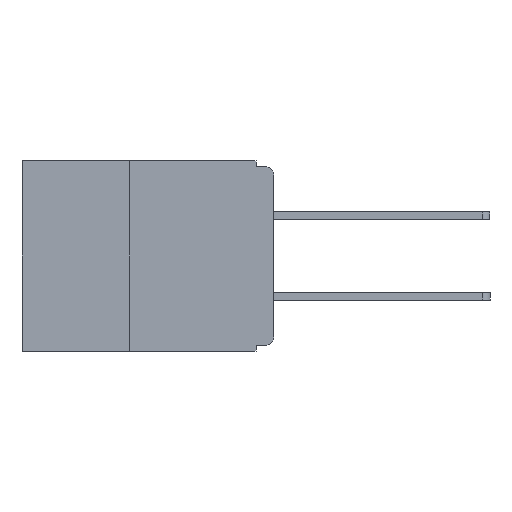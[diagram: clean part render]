
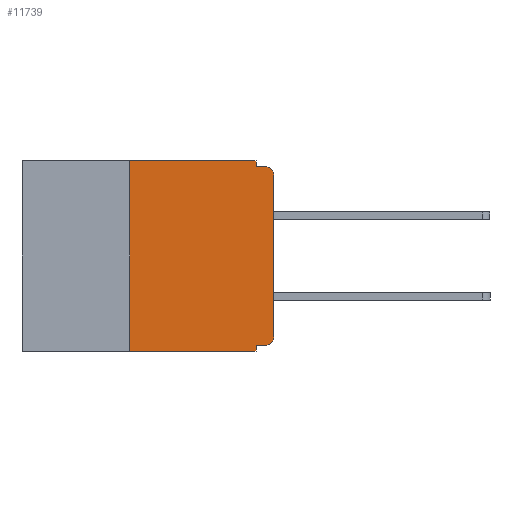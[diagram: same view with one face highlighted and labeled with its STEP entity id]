
A CAD part, left-side view. The second image highlights one B-rep face of the part: STEP entity #11739.
In plain terms, the highlighted planar face has unit normal (-1, 0, 0).
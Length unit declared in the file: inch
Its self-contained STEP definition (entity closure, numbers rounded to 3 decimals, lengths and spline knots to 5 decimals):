
#386 = CARTESIAN_POINT ( 'NONE',  ( 0., 0., -0.305 ) ) ;
#990 = VERTEX_POINT ( 'NONE', #12404 ) ;
#1145 = VERTEX_POINT ( 'NONE', #3089 ) ;
#1475 = LINE ( 'NONE', #6721, #4894 ) ;
#1728 = ORIENTED_EDGE ( 'NONE', *, *, #4678, .T. ) ;
#1759 = EDGE_CURVE ( 'NONE', #8024, #1145, #12991, .T. ) ;
#1938 = EDGE_CURVE ( 'NONE', #990, #3292, #2088, .T. ) ;
#2088 = LINE ( 'NONE', #8318, #7469 ) ;
#2094 = ORIENTED_EDGE ( 'NONE', *, *, #13673, .T. ) ;
#2218 = LINE ( 'NONE', #14178, #7942 ) ;
#2432 = ORIENTED_EDGE ( 'NONE', *, *, #4056, .F. ) ;
#2573 = CARTESIAN_POINT ( 'NONE',  ( 0., 0.437, 0. ) ) ;
#2944 = DIRECTION ( 'NONE',  ( -1., 0., 0. ) ) ;
#2991 = ORIENTED_EDGE ( 'NONE', *, *, #1938, .F. ) ;
#3089 = CARTESIAN_POINT ( 'NONE',  ( 0., 0.031, -0.33 ) ) ;
#3232 = CARTESIAN_POINT ( 'NONE',  ( 0., 0.015, -0.305 ) ) ;
#3292 = VERTEX_POINT ( 'NONE', #6554 ) ;
#3412 = ORIENTED_EDGE ( 'NONE', *, *, #3512, .F. ) ;
#3512 = EDGE_CURVE ( 'NONE', #6207, #990, #2218, .T. ) ;
#3688 = EDGE_CURVE ( 'NONE', #4758, #1145, #11585, .T. ) ;
#3736 = DIRECTION ( 'NONE',  ( 0., 0., -1. ) ) ;
#3903 = VECTOR ( 'NONE', #8673, 39.37008 ) ;
#4056 = EDGE_CURVE ( 'NONE', #3292, #9083, #5090, .T. ) ;
#4080 = AXIS2_PLACEMENT_3D ( 'NONE', #9697, #2944, #10752 ) ;
#4146 = ORIENTED_EDGE ( 'NONE', *, *, #6434, .F. ) ;
#4300 = AXIS2_PLACEMENT_3D ( 'NONE', #3232, #11186, #4588 ) ;
#4315 = CARTESIAN_POINT ( 'NONE',  ( 0., 0.437, -0.33 ) ) ;
#4477 = ORIENTED_EDGE ( 'NONE', *, *, #1759, .T. ) ;
#4588 = DIRECTION ( 'NONE',  ( 0., 0., -1. ) ) ;
#4678 = EDGE_CURVE ( 'NONE', #6570, #8162, #1475, .T. ) ;
#4758 = VERTEX_POINT ( 'NONE', #6008 ) ;
#4894 = VECTOR ( 'NONE', #6567, 39.37008 ) ;
#5090 = LINE ( 'NONE', #11175, #10291 ) ;
#5576 = ORIENTED_EDGE ( 'NONE', *, *, #3688, .F. ) ;
#5739 = ORIENTED_EDGE ( 'NONE', *, *, #8268, .F. ) ;
#5898 = CARTESIAN_POINT ( 'NONE',  ( 0., 0., -0.32 ) ) ;
#6008 = CARTESIAN_POINT ( 'NONE',  ( 0., 0.031, -0.32 ) ) ;
#6207 = VERTEX_POINT ( 'NONE', #8849 ) ;
#6264 = LINE ( 'NONE', #10243, #14175 ) ;
#6353 = ORIENTED_EDGE ( 'NONE', *, *, #8973, .T. ) ;
#6434 = EDGE_CURVE ( 'NONE', #8024, #6207, #6264, .T. ) ;
#6554 = CARTESIAN_POINT ( 'NONE',  ( 0., 0.031, -0.01 ) ) ;
#6567 = DIRECTION ( 'NONE',  ( 0., 0., 1. ) ) ;
#6570 = VERTEX_POINT ( 'NONE', #386 ) ;
#6721 = CARTESIAN_POINT ( 'NONE',  ( 0., 0., 0. ) ) ;
#6853 = FACE_OUTER_BOUND ( 'NONE', #13814, .T. ) ;
#7123 = PLANE ( 'NONE',  #13590 ) ;
#7469 = VECTOR ( 'NONE', #12516, 39.37008 ) ;
#7942 = VECTOR ( 'NONE', #14147, 39.37008 ) ;
#8024 = VERTEX_POINT ( 'NONE', #8566 ) ;
#8042 = LINE ( 'NONE', #5898, #13371 ) ;
#8162 = VERTEX_POINT ( 'NONE', #11160 ) ;
#8185 = DIRECTION ( 'NONE',  ( 0., 1., 0. ) ) ;
#8268 = EDGE_CURVE ( 'NONE', #11644, #4758, #8042, .T. ) ;
#8318 = CARTESIAN_POINT ( 'NONE',  ( 0., 0.031, 0. ) ) ;
#8566 = CARTESIAN_POINT ( 'NONE',  ( 0., 0.25, -0.33 ) ) ;
#8673 = DIRECTION ( 'NONE',  ( 0., -1., 0. ) ) ;
#8849 = CARTESIAN_POINT ( 'NONE',  ( 0., 0.25, 0. ) ) ;
#8973 = EDGE_CURVE ( 'NONE', #11644, #6570, #13523, .T. ) ;
#9083 = VERTEX_POINT ( 'NONE', #10323 ) ;
#9697 = CARTESIAN_POINT ( 'NONE',  ( 0., 0.015, -0.025 ) ) ;
#9734 = CIRCLE ( 'NONE', #4080, 0.015 ) ;
#10243 = CARTESIAN_POINT ( 'NONE',  ( 0., 0.25, -0.33 ) ) ;
#10291 = VECTOR ( 'NONE', #11169, 39.37008 ) ;
#10323 = CARTESIAN_POINT ( 'NONE',  ( 0., 0.015, -0.01 ) ) ;
#10387 = DIRECTION ( 'NONE',  ( 1., 0., 0. ) ) ;
#10752 = DIRECTION ( 'NONE',  ( 0., 0., -1. ) ) ;
#11160 = CARTESIAN_POINT ( 'NONE',  ( 0., 0., -0.025 ) ) ;
#11169 = DIRECTION ( 'NONE',  ( 0., -1., 0. ) ) ;
#11175 = CARTESIAN_POINT ( 'NONE',  ( 0., 0., -0.01 ) ) ;
#11186 = DIRECTION ( 'NONE',  ( -1., 0., 0. ) ) ;
#11249 = VECTOR ( 'NONE', #13141, 39.37008 ) ;
#11585 = LINE ( 'NONE', #13146, #11249 ) ;
#11644 = VERTEX_POINT ( 'NONE', #13409 ) ;
#11739 = ADVANCED_FACE ( 'NONE', ( #6853 ), #7123, .F. ) ;
#12404 = CARTESIAN_POINT ( 'NONE',  ( 0., 0.031, 0. ) ) ;
#12516 = DIRECTION ( 'NONE',  ( 0., 0., -1. ) ) ;
#12991 = LINE ( 'NONE', #4315, #3903 ) ;
#13141 = DIRECTION ( 'NONE',  ( 0., 0., -1. ) ) ;
#13146 = CARTESIAN_POINT ( 'NONE',  ( 0., 0.031, -0.33 ) ) ;
#13371 = VECTOR ( 'NONE', #8185, 39.37008 ) ;
#13409 = CARTESIAN_POINT ( 'NONE',  ( 0., 0.015, -0.32 ) ) ;
#13451 = DIRECTION ( 'NONE',  ( 0., 0., 1. ) ) ;
#13523 = CIRCLE ( 'NONE', #4300, 0.015 ) ;
#13590 = AXIS2_PLACEMENT_3D ( 'NONE', #2573, #10387, #3736 ) ;
#13673 = EDGE_CURVE ( 'NONE', #8162, #9083, #9734, .T. ) ;
#13814 = EDGE_LOOP ( 'NONE', ( #1728, #2094, #2432, #2991, #3412, #4146, #4477, #5576, #5739, #6353 ) ) ;
#14147 = DIRECTION ( 'NONE',  ( 0., -1., 0. ) ) ;
#14175 = VECTOR ( 'NONE', #13451, 39.37008 ) ;
#14178 = CARTESIAN_POINT ( 'NONE',  ( 0., 0.437, 0. ) ) ;
